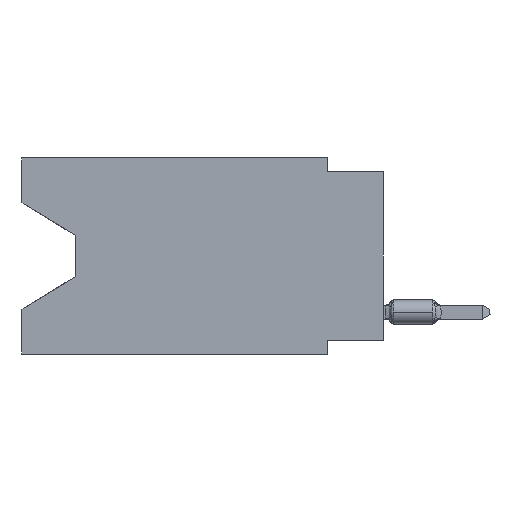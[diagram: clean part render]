
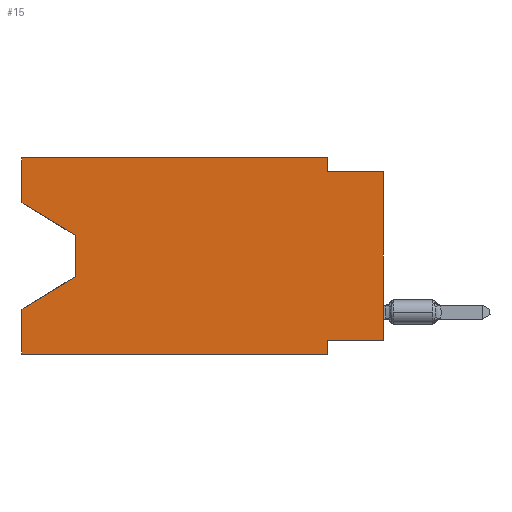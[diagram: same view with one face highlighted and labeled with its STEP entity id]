
A CAD part, left-side view. The second image highlights one B-rep face of the part: STEP entity #15.
In plain terms, the highlighted planar face has unit normal (-1, 0, 0).
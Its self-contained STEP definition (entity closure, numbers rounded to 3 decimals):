
#15 = ADVANCED_FACE ( 'NONE', ( #62659 ), #9846, .F. ) ;
#801 = VECTOR ( 'NONE', #38682, 1000. ) ;
#853 = VERTEX_POINT ( 'NONE', #22187 ) ;
#2199 = LINE ( 'NONE', #21725, #41447 ) ;
#2867 = LINE ( 'NONE', #31672, #30867 ) ;
#3372 = CARTESIAN_POINT ( 'NONE',  ( 0., 2.54, -0.635 ) ) ;
#3816 = CARTESIAN_POINT ( 'NONE',  ( 0., 2.54, -8.89 ) ) ;
#4248 = EDGE_CURVE ( 'NONE', #18295, #57859, #62636, .T. ) ;
#5034 = DIRECTION ( 'NONE',  ( 0., 0., -1. ) ) ;
#5350 = EDGE_CURVE ( 'NONE', #5777, #57859, #21396, .T. ) ;
#5559 = CARTESIAN_POINT ( 'NONE',  ( 0., 0., -0.635 ) ) ;
#5777 = VERTEX_POINT ( 'NONE', #61012 ) ;
#6546 = EDGE_CURVE ( 'NONE', #62831, #45382, #21533, .T. ) ;
#7525 = VECTOR ( 'NONE', #42918, 1000. ) ;
#9192 = DIRECTION ( 'NONE',  ( 0., 0., -1. ) ) ;
#9846 = PLANE ( 'NONE',  #13095 ) ;
#10474 = LINE ( 'NONE', #30014, #47160 ) ;
#11436 = CARTESIAN_POINT ( 'NONE',  ( 0., 0., -0.635 ) ) ;
#12808 = EDGE_CURVE ( 'NONE', #853, #5777, #2867, .T. ) ;
#13024 = VERTEX_POINT ( 'NONE', #3816 ) ;
#13095 = AXIS2_PLACEMENT_3D ( 'NONE', #19422, #43129, #9192 ) ;
#13179 = DIRECTION ( 'NONE',  ( 0., 1., 0. ) ) ;
#13541 = DIRECTION ( 'NONE',  ( 0., -1., 0. ) ) ;
#13696 = ORIENTED_EDGE ( 'NONE', *, *, #45876, .T. ) ;
#14642 = VERTEX_POINT ( 'NONE', #18380 ) ;
#14698 = ORIENTED_EDGE ( 'NONE', *, *, #12808, .T. ) ;
#15654 = CARTESIAN_POINT ( 'NONE',  ( 0., 13.97, -5.385 ) ) ;
#15908 = ORIENTED_EDGE ( 'NONE', *, *, #42983, .F. ) ;
#16847 = ORIENTED_EDGE ( 'NONE', *, *, #40394, .T. ) ;
#17198 = ORIENTED_EDGE ( 'NONE', *, *, #53703, .F. ) ;
#18295 = VERTEX_POINT ( 'NONE', #59409 ) ;
#18380 = CARTESIAN_POINT ( 'NONE',  ( 0., 2.54, 0. ) ) ;
#19422 = CARTESIAN_POINT ( 'NONE',  ( 0., 16.383, 0. ) ) ;
#19939 = EDGE_CURVE ( 'NONE', #45382, #13024, #42478, .T. ) ;
#20695 = VERTEX_POINT ( 'NONE', #5559 ) ;
#21207 = ORIENTED_EDGE ( 'NONE', *, *, #58118, .T. ) ;
#21396 = LINE ( 'NONE', #15654, #31998 ) ;
#21533 = LINE ( 'NONE', #26976, #44276 ) ;
#21610 = ORIENTED_EDGE ( 'NONE', *, *, #26371, .F. ) ;
#21670 = EDGE_CURVE ( 'NONE', #29713, #14642, #24924, .T. ) ;
#21707 = EDGE_LOOP ( 'NONE', ( #13696, #14698, #36131, #47409, #16847, #29832, #59874, #21207, #21610, #15908, #43577, #17198 ) ) ;
#21725 = CARTESIAN_POINT ( 'NONE',  ( 0., 16.383, -2.038 ) ) ;
#22187 = CARTESIAN_POINT ( 'NONE',  ( 0., 13.97, -3.505 ) ) ;
#22311 = DIRECTION ( 'NONE',  ( 0., 0., -1. ) ) ;
#23386 = LINE ( 'NONE', #33322, #7525 ) ;
#24101 = VECTOR ( 'NONE', #30964, 1000. ) ;
#24924 = LINE ( 'NONE', #29724, #801 ) ;
#26371 = EDGE_CURVE ( 'NONE', #55887, #20695, #55289, .T. ) ;
#26512 = DIRECTION ( 'NONE',  ( 0., 0.855, -0.519 ) ) ;
#26976 = CARTESIAN_POINT ( 'NONE',  ( 0., 0., -8.255 ) ) ;
#27046 = CARTESIAN_POINT ( 'NONE',  ( 0., 16.383, -2.038 ) ) ;
#27118 = CARTESIAN_POINT ( 'NONE',  ( 0., 2.54, -8.89 ) ) ;
#27237 = LINE ( 'NONE', #32347, #56326 ) ;
#27547 = DIRECTION ( 'NONE',  ( 0., 0., 1. ) ) ;
#29713 = VERTEX_POINT ( 'NONE', #32379 ) ;
#29724 = CARTESIAN_POINT ( 'NONE',  ( 0., 16.383, 0. ) ) ;
#29832 = ORIENTED_EDGE ( 'NONE', *, *, #19939, .F. ) ;
#30014 = CARTESIAN_POINT ( 'NONE',  ( 0., 2.54, 0. ) ) ;
#30867 = VECTOR ( 'NONE', #31989, 1000. ) ;
#30964 = DIRECTION ( 'NONE',  ( 0., -1., 0. ) ) ;
#31672 = CARTESIAN_POINT ( 'NONE',  ( 0., 13.97, -3.505 ) ) ;
#31701 = CARTESIAN_POINT ( 'NONE',  ( 0., 2.54, -8.255 ) ) ;
#31989 = DIRECTION ( 'NONE',  ( 0., 0., -1. ) ) ;
#31998 = VECTOR ( 'NONE', #26512, 1000. ) ;
#32347 = CARTESIAN_POINT ( 'NONE',  ( 0., 16.383, 0. ) ) ;
#32379 = CARTESIAN_POINT ( 'NONE',  ( 0., 16.383, 0. ) ) ;
#33322 = CARTESIAN_POINT ( 'NONE',  ( 0., 0., 0. ) ) ;
#33882 = CARTESIAN_POINT ( 'NONE',  ( 0., 0., -8.255 ) ) ;
#36131 = ORIENTED_EDGE ( 'NONE', *, *, #5350, .T. ) ;
#38527 = CARTESIAN_POINT ( 'NONE',  ( 0., 16.383, -8.89 ) ) ;
#38682 = DIRECTION ( 'NONE',  ( 0., -1., 0. ) ) ;
#39386 = VERTEX_POINT ( 'NONE', #27046 ) ;
#40394 = EDGE_CURVE ( 'NONE', #18295, #13024, #43335, .T. ) ;
#40735 = CARTESIAN_POINT ( 'NONE',  ( 0., 16.383, -6.852 ) ) ;
#41125 = VECTOR ( 'NONE', #43984, 1000. ) ;
#41265 = DIRECTION ( 'NONE',  ( 0., -0.855, -0.519 ) ) ;
#41447 = VECTOR ( 'NONE', #41265, 1000. ) ;
#42478 = LINE ( 'NONE', #27118, #49691 ) ;
#42918 = DIRECTION ( 'NONE',  ( 0., 0., 1. ) ) ;
#42983 = EDGE_CURVE ( 'NONE', #14642, #55887, #10474, .T. ) ;
#43129 = DIRECTION ( 'NONE',  ( 1., 0., 0. ) ) ;
#43335 = LINE ( 'NONE', #38527, #58636 ) ;
#43577 = ORIENTED_EDGE ( 'NONE', *, *, #21670, .F. ) ;
#43984 = DIRECTION ( 'NONE',  ( 0., 0., 1. ) ) ;
#44276 = VECTOR ( 'NONE', #13179, 1000. ) ;
#45382 = VERTEX_POINT ( 'NONE', #31701 ) ;
#45876 = EDGE_CURVE ( 'NONE', #39386, #853, #2199, .T. ) ;
#47160 = VECTOR ( 'NONE', #5034, 1000. ) ;
#47409 = ORIENTED_EDGE ( 'NONE', *, *, #4248, .F. ) ;
#49691 = VECTOR ( 'NONE', #22311, 1000. ) ;
#53703 = EDGE_CURVE ( 'NONE', #39386, #29713, #27237, .T. ) ;
#53910 = CARTESIAN_POINT ( 'NONE',  ( 0., 16.383, 0. ) ) ;
#55289 = LINE ( 'NONE', #11436, #24101 ) ;
#55887 = VERTEX_POINT ( 'NONE', #3372 ) ;
#56326 = VECTOR ( 'NONE', #27547, 1000. ) ;
#57859 = VERTEX_POINT ( 'NONE', #40735 ) ;
#58118 = EDGE_CURVE ( 'NONE', #62831, #20695, #23386, .T. ) ;
#58636 = VECTOR ( 'NONE', #13541, 1000. ) ;
#59409 = CARTESIAN_POINT ( 'NONE',  ( 0., 16.383, -8.89 ) ) ;
#59874 = ORIENTED_EDGE ( 'NONE', *, *, #6546, .F. ) ;
#61012 = CARTESIAN_POINT ( 'NONE',  ( 0., 13.97, -5.385 ) ) ;
#62636 = LINE ( 'NONE', #53910, #41125 ) ;
#62659 = FACE_OUTER_BOUND ( 'NONE', #21707, .T. ) ;
#62831 = VERTEX_POINT ( 'NONE', #33882 ) ;
